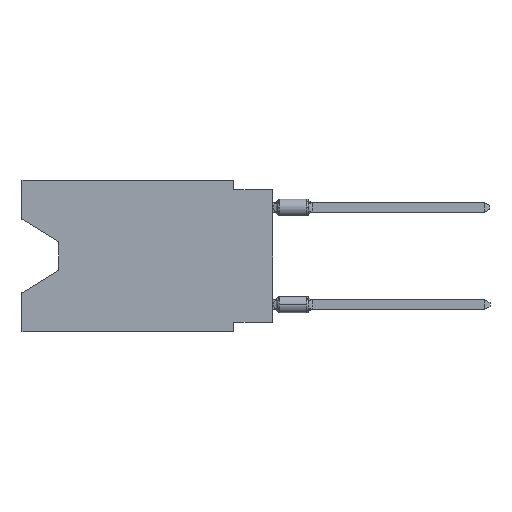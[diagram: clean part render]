
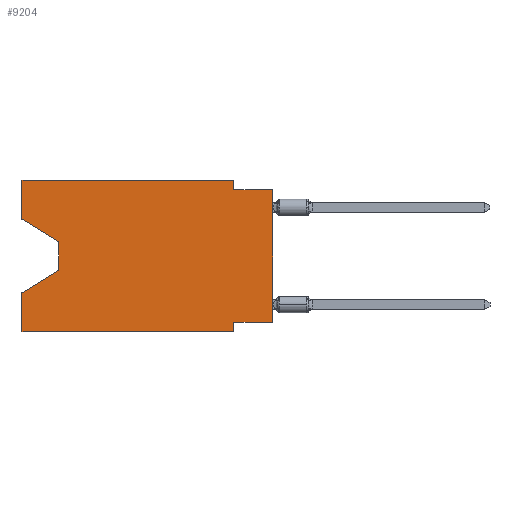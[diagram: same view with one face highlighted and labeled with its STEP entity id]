
A CAD part, left-side view. The second image highlights one B-rep face of the part: STEP entity #9204.
In plain terms, the highlighted planar face has unit normal (-1, 0, 0).
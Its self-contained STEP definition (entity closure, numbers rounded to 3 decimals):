
#56 = LINE ( 'NONE', #16049, #18345 ) ;
#151 = CARTESIAN_POINT ( 'NONE',  ( 0., 16.383, -9.906 ) ) ;
#162 = CARTESIAN_POINT ( 'NONE',  ( 0., 13.97, -5.893 ) ) ;
#186 = EDGE_CURVE ( 'NONE', #6610, #243, #18500, .T. ) ;
#232 = VERTEX_POINT ( 'NONE', #162 ) ;
#243 = VERTEX_POINT ( 'NONE', #1297 ) ;
#458 = LINE ( 'NONE', #6209, #8649 ) ;
#492 = VECTOR ( 'NONE', #5638, 1000. ) ;
#500 = LINE ( 'NONE', #3603, #13803 ) ;
#608 = ORIENTED_EDGE ( 'NONE', *, *, #17327, .F. ) ;
#649 = VERTEX_POINT ( 'NONE', #15577 ) ;
#716 = VECTOR ( 'NONE', #7613, 1000. ) ;
#887 = ORIENTED_EDGE ( 'NONE', *, *, #15407, .F. ) ;
#1175 = ORIENTED_EDGE ( 'NONE', *, *, #12593, .F. ) ;
#1289 = LINE ( 'NONE', #8435, #2188 ) ;
#1296 = CARTESIAN_POINT ( 'NONE',  ( 0., 0., -9.271 ) ) ;
#1297 = CARTESIAN_POINT ( 'NONE',  ( 0., 2.54, -9.906 ) ) ;
#1475 = DIRECTION ( 'NONE',  ( 0., 0., -1. ) ) ;
#1560 = DIRECTION ( 'NONE',  ( 0., 0., 1. ) ) ;
#1702 = DIRECTION ( 'NONE',  ( 0., 0., 1. ) ) ;
#1782 = LINE ( 'NONE', #1872, #716 ) ;
#1797 = CARTESIAN_POINT ( 'NONE',  ( 0., 16.383, 0. ) ) ;
#1872 = CARTESIAN_POINT ( 'NONE',  ( 0., 13.97, -4.013 ) ) ;
#2002 = VECTOR ( 'NONE', #12219, 1000. ) ;
#2188 = VECTOR ( 'NONE', #1475, 1000. ) ;
#2548 = EDGE_CURVE ( 'NONE', #12371, #4164, #9907, .T. ) ;
#2645 = DIRECTION ( 'NONE',  ( 0., 0., -1. ) ) ;
#2731 = CARTESIAN_POINT ( 'NONE',  ( 0., 2.54, -0.635 ) ) ;
#2755 = DIRECTION ( 'NONE',  ( 0., -0.855, -0.519 ) ) ;
#3006 = LINE ( 'NONE', #1797, #14029 ) ;
#3274 = EDGE_CURVE ( 'NONE', #18583, #18297, #56, .T. ) ;
#3589 = CARTESIAN_POINT ( 'NONE',  ( 0., 2.54, 0. ) ) ;
#3603 = CARTESIAN_POINT ( 'NONE',  ( 0., 13.97, -5.893 ) ) ;
#3672 = DIRECTION ( 'NONE',  ( 0., 1., 0. ) ) ;
#4164 = VERTEX_POINT ( 'NONE', #8763 ) ;
#4310 = CARTESIAN_POINT ( 'NONE',  ( 0., 16.383, 0. ) ) ;
#4939 = ORIENTED_EDGE ( 'NONE', *, *, #17414, .F. ) ;
#5034 = EDGE_CURVE ( 'NONE', #6610, #18308, #6213, .T. ) ;
#5068 = VERTEX_POINT ( 'NONE', #17844 ) ;
#5570 = CARTESIAN_POINT ( 'NONE',  ( 0., 16.383, 0. ) ) ;
#5638 = DIRECTION ( 'NONE',  ( 0., -1., 0. ) ) ;
#5845 = VERTEX_POINT ( 'NONE', #3589 ) ;
#6209 = CARTESIAN_POINT ( 'NONE',  ( 0., 2.54, -9.906 ) ) ;
#6213 = LINE ( 'NONE', #11950, #2002 ) ;
#6610 = VERTEX_POINT ( 'NONE', #151 ) ;
#7180 = DIRECTION ( 'NONE',  ( 0., -1., 0. ) ) ;
#7248 = PLANE ( 'NONE',  #13519 ) ;
#7613 = DIRECTION ( 'NONE',  ( 0., 0., -1. ) ) ;
#7745 = ORIENTED_EDGE ( 'NONE', *, *, #10994, .F. ) ;
#7903 = CARTESIAN_POINT ( 'NONE',  ( 0., 16.383, -7.36 ) ) ;
#8006 = ORIENTED_EDGE ( 'NONE', *, *, #186, .T. ) ;
#8380 = DIRECTION ( 'NONE',  ( 1., 0., 0. ) ) ;
#8435 = CARTESIAN_POINT ( 'NONE',  ( 0., 2.54, 0. ) ) ;
#8649 = VECTOR ( 'NONE', #11945, 1000. ) ;
#8763 = CARTESIAN_POINT ( 'NONE',  ( 0., 13.97, -4.013 ) ) ;
#8873 = LINE ( 'NONE', #9651, #10980 ) ;
#8922 = EDGE_CURVE ( 'NONE', #232, #18308, #500, .T. ) ;
#9204 = ADVANCED_FACE ( 'NONE', ( #15897 ), #7248, .F. ) ;
#9231 = CARTESIAN_POINT ( 'NONE',  ( 0., 0., -0.635 ) ) ;
#9651 = CARTESIAN_POINT ( 'NONE',  ( 0., 0., -0.635 ) ) ;
#9712 = EDGE_LOOP ( 'NONE', ( #12446, #18077, #17920, #18004, #8006, #7745, #887, #12533, #1175, #608, #4939, #15736 ) ) ;
#9907 = LINE ( 'NONE', #15641, #11420 ) ;
#10740 = CARTESIAN_POINT ( 'NONE',  ( 0., 0., -9.271 ) ) ;
#10980 = VECTOR ( 'NONE', #7180, 1000. ) ;
#10994 = EDGE_CURVE ( 'NONE', #649, #243, #458, .T. ) ;
#11420 = VECTOR ( 'NONE', #2755, 1000. ) ;
#11945 = DIRECTION ( 'NONE',  ( 0., 0., -1. ) ) ;
#11950 = CARTESIAN_POINT ( 'NONE',  ( 0., 16.383, 0. ) ) ;
#12067 = VERTEX_POINT ( 'NONE', #2731 ) ;
#12077 = DIRECTION ( 'NONE',  ( 0., 0.855, -0.519 ) ) ;
#12219 = DIRECTION ( 'NONE',  ( 0., 0., 1. ) ) ;
#12320 = LINE ( 'NONE', #10740, #13637 ) ;
#12371 = VERTEX_POINT ( 'NONE', #15515 ) ;
#12446 = ORIENTED_EDGE ( 'NONE', *, *, #2548, .T. ) ;
#12533 = ORIENTED_EDGE ( 'NONE', *, *, #3274, .T. ) ;
#12593 = EDGE_CURVE ( 'NONE', #12067, #18297, #8873, .T. ) ;
#12957 = DIRECTION ( 'NONE',  ( 0., -1., 0. ) ) ;
#13053 = LINE ( 'NONE', #4310, #492 ) ;
#13519 = AXIS2_PLACEMENT_3D ( 'NONE', #5570, #8380, #2645 ) ;
#13637 = VECTOR ( 'NONE', #3672, 1000. ) ;
#13803 = VECTOR ( 'NONE', #12077, 1000. ) ;
#14029 = VECTOR ( 'NONE', #1702, 1000. ) ;
#14189 = CARTESIAN_POINT ( 'NONE',  ( 0., 16.383, -9.906 ) ) ;
#15407 = EDGE_CURVE ( 'NONE', #18583, #649, #12320, .T. ) ;
#15448 = VECTOR ( 'NONE', #12957, 1000. ) ;
#15515 = CARTESIAN_POINT ( 'NONE',  ( 0., 16.383, -2.546 ) ) ;
#15577 = CARTESIAN_POINT ( 'NONE',  ( 0., 2.54, -9.271 ) ) ;
#15641 = CARTESIAN_POINT ( 'NONE',  ( 0., 16.383, -2.546 ) ) ;
#15697 = EDGE_CURVE ( 'NONE', #4164, #232, #1782, .T. ) ;
#15736 = ORIENTED_EDGE ( 'NONE', *, *, #18219, .F. ) ;
#15897 = FACE_OUTER_BOUND ( 'NONE', #9712, .T. ) ;
#16049 = CARTESIAN_POINT ( 'NONE',  ( 0., 0., 0. ) ) ;
#17327 = EDGE_CURVE ( 'NONE', #5845, #12067, #1289, .T. ) ;
#17414 = EDGE_CURVE ( 'NONE', #5068, #5845, #13053, .T. ) ;
#17844 = CARTESIAN_POINT ( 'NONE',  ( 0., 16.383, 0. ) ) ;
#17920 = ORIENTED_EDGE ( 'NONE', *, *, #8922, .T. ) ;
#18004 = ORIENTED_EDGE ( 'NONE', *, *, #5034, .F. ) ;
#18077 = ORIENTED_EDGE ( 'NONE', *, *, #15697, .T. ) ;
#18219 = EDGE_CURVE ( 'NONE', #12371, #5068, #3006, .T. ) ;
#18297 = VERTEX_POINT ( 'NONE', #9231 ) ;
#18308 = VERTEX_POINT ( 'NONE', #7903 ) ;
#18345 = VECTOR ( 'NONE', #1560, 1000. ) ;
#18500 = LINE ( 'NONE', #14189, #15448 ) ;
#18583 = VERTEX_POINT ( 'NONE', #1296 ) ;
